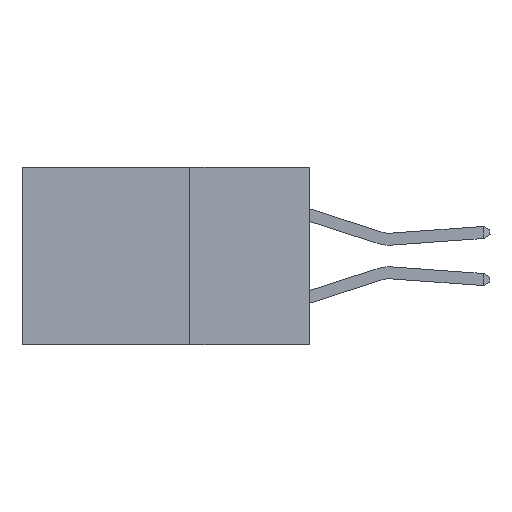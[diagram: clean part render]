
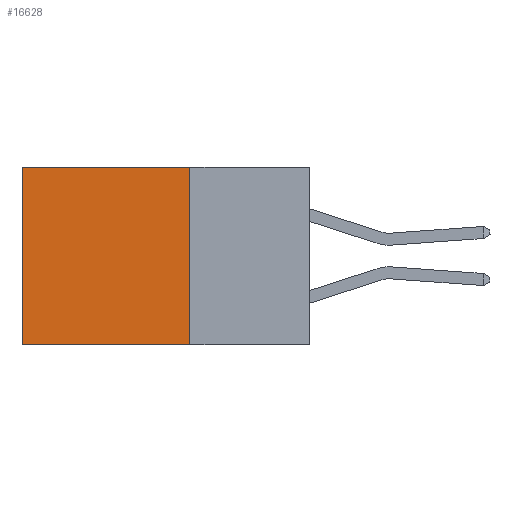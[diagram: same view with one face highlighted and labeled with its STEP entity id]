
A CAD part, left-side view. The second image highlights one B-rep face of the part: STEP entity #16628.
In plain terms, the highlighted planar face has unit normal (-1, 0, 0).
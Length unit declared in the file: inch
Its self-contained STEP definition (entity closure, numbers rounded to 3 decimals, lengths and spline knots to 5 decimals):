
#2849 = EDGE_CURVE ( 'NONE', #19204, #19097, #8244, .T. ) ;
#3478 = ORIENTED_EDGE ( 'NONE', *, *, #2849, .F. ) ;
#4799 = PLANE ( 'NONE',  #23739 ) ;
#5882 = CARTESIAN_POINT ( 'NONE',  ( 0.298, 0.25, 0. ) ) ;
#6195 = EDGE_CURVE ( 'NONE', #24290, #8117, #25561, .T. ) ;
#6227 = LINE ( 'NONE', #25841, #17155 ) ;
#6639 = FACE_OUTER_BOUND ( 'NONE', #15774, .T. ) ;
#6748 = ORIENTED_EDGE ( 'NONE', *, *, #8150, .F. ) ;
#7016 = CARTESIAN_POINT ( 'NONE',  ( 0.298, 0.25, 0. ) ) ;
#7528 = VECTOR ( 'NONE', #10127, 39.37008 ) ;
#8117 = VERTEX_POINT ( 'NONE', #18507 ) ;
#8150 = EDGE_CURVE ( 'NONE', #24290, #19204, #22440, .T. ) ;
#8244 = LINE ( 'NONE', #10800, #7528 ) ;
#8762 = ORIENTED_EDGE ( 'NONE', *, *, #6195, .T. ) ;
#10127 = DIRECTION ( 'NONE',  ( 0., 1., 0. ) ) ;
#10800 = CARTESIAN_POINT ( 'NONE',  ( 0.298, 0.25, -0.37 ) ) ;
#11472 = DIRECTION ( 'NONE',  ( 0., 0., -1. ) ) ;
#15774 = EDGE_LOOP ( 'NONE', ( #19418, #3478, #6748, #8762 ) ) ;
#16628 = ADVANCED_FACE ( 'NONE', ( #6639 ), #4799, .F. ) ;
#16925 = CARTESIAN_POINT ( 'NONE',  ( 0.298, 0.25, 0. ) ) ;
#17155 = VECTOR ( 'NONE', #27984, 39.37008 ) ;
#17591 = CARTESIAN_POINT ( 'NONE',  ( 0.298, 0.25, -0.37 ) ) ;
#18507 = CARTESIAN_POINT ( 'NONE',  ( 0.298, 0.6, 0. ) ) ;
#19010 = DIRECTION ( 'NONE',  ( 0., 1., 0. ) ) ;
#19097 = VERTEX_POINT ( 'NONE', #21497 ) ;
#19204 = VERTEX_POINT ( 'NONE', #17591 ) ;
#19418 = ORIENTED_EDGE ( 'NONE', *, *, #25798, .T. ) ;
#20534 = VECTOR ( 'NONE', #19010, 39.37008 ) ;
#21497 = CARTESIAN_POINT ( 'NONE',  ( 0.298, 0.6, -0.37 ) ) ;
#22440 = LINE ( 'NONE', #22863, #27439 ) ;
#22863 = CARTESIAN_POINT ( 'NONE',  ( 0.298, 0.25, 0. ) ) ;
#23739 = AXIS2_PLACEMENT_3D ( 'NONE', #7016, #24307, #11472 ) ;
#24290 = VERTEX_POINT ( 'NONE', #16925 ) ;
#24307 = DIRECTION ( 'NONE',  ( 1., 0., 0. ) ) ;
#25027 = DIRECTION ( 'NONE',  ( 0., 0., -1. ) ) ;
#25561 = LINE ( 'NONE', #5882, #20534 ) ;
#25798 = EDGE_CURVE ( 'NONE', #8117, #19097, #6227, .T. ) ;
#25841 = CARTESIAN_POINT ( 'NONE',  ( 0.298, 0.6, 0. ) ) ;
#27439 = VECTOR ( 'NONE', #25027, 39.37008 ) ;
#27984 = DIRECTION ( 'NONE',  ( 0., 0., -1. ) ) ;
